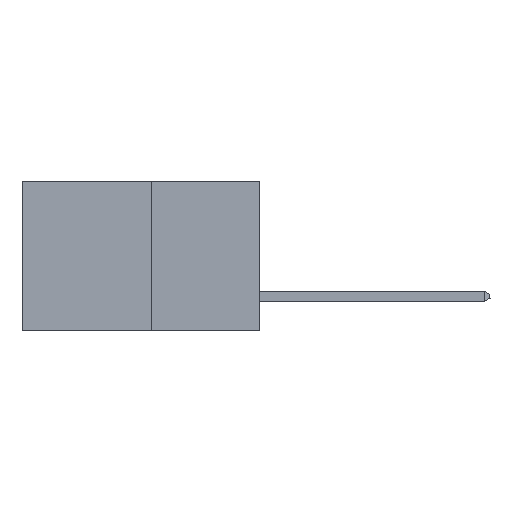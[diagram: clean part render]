
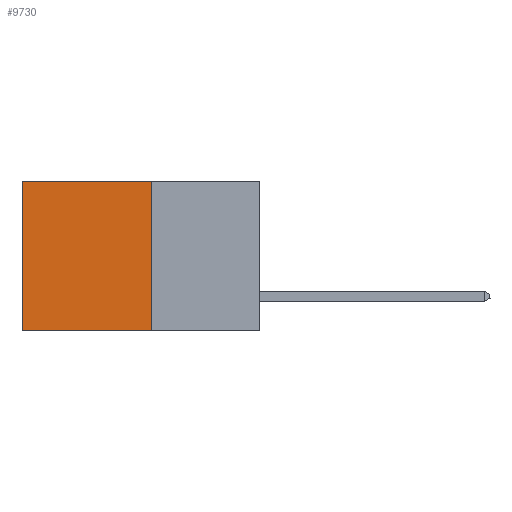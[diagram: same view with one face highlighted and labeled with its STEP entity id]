
A CAD part, left-side view. The second image highlights one B-rep face of the part: STEP entity #9730.
In plain terms, the highlighted planar face has unit normal (-1, 0, 0).
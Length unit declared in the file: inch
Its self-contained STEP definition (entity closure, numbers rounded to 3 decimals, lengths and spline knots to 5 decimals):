
#155 = DIRECTION ( 'NONE',  ( 0., 1., 0. ) ) ;
#170 = VERTEX_POINT ( 'NONE', #330 ) ;
#330 = CARTESIAN_POINT ( 'NONE',  ( 0.277, 0.59, -0.37 ) ) ;
#566 = FACE_OUTER_BOUND ( 'NONE', #10602, .T. ) ;
#955 = VECTOR ( 'NONE', #10435, 39.37008 ) ;
#1531 = LINE ( 'NONE', #7736, #13517 ) ;
#1751 = CARTESIAN_POINT ( 'NONE',  ( 0.277, 0.59, 0. ) ) ;
#1821 = ORIENTED_EDGE ( 'NONE', *, *, #8032, .T. ) ;
#2456 = EDGE_CURVE ( 'NONE', #14388, #170, #10186, .T. ) ;
#2959 = CARTESIAN_POINT ( 'NONE',  ( 0.277, 0.27, -0.37 ) ) ;
#2979 = DIRECTION ( 'NONE',  ( 0., 1., 0. ) ) ;
#3115 = LINE ( 'NONE', #12304, #8902 ) ;
#3394 = VERTEX_POINT ( 'NONE', #14742 ) ;
#3771 = VERTEX_POINT ( 'NONE', #8784 ) ;
#3879 = ORIENTED_EDGE ( 'NONE', *, *, #10291, .F. ) ;
#3886 = CARTESIAN_POINT ( 'NONE',  ( 0.277, 0.27, -0.37 ) ) ;
#5059 = DIRECTION ( 'NONE',  ( 0., 0., -1. ) ) ;
#5264 = VECTOR ( 'NONE', #5059, 39.37008 ) ;
#5602 = ORIENTED_EDGE ( 'NONE', *, *, #2456, .T. ) ;
#6443 = PLANE ( 'NONE',  #7658 ) ;
#7596 = DIRECTION ( 'NONE',  ( 0., 0., -1. ) ) ;
#7658 = AXIS2_PLACEMENT_3D ( 'NONE', #2959, #14531, #7596 ) ;
#7736 = CARTESIAN_POINT ( 'NONE',  ( 0.277, 0.27, 0. ) ) ;
#8032 = EDGE_CURVE ( 'NONE', #3394, #14388, #1531, .T. ) ;
#8784 = CARTESIAN_POINT ( 'NONE',  ( 0.277, 0.27, -0.37 ) ) ;
#8902 = VECTOR ( 'NONE', #2979, 39.37008 ) ;
#9730 = ADVANCED_FACE ( 'NONE', ( #566 ), #6443, .F. ) ;
#10186 = LINE ( 'NONE', #10895, #955 ) ;
#10203 = ORIENTED_EDGE ( 'NONE', *, *, #11891, .F. ) ;
#10291 = EDGE_CURVE ( 'NONE', #3394, #3771, #11477, .T. ) ;
#10435 = DIRECTION ( 'NONE',  ( 0., 0., -1. ) ) ;
#10602 = EDGE_LOOP ( 'NONE', ( #5602, #10203, #3879, #1821 ) ) ;
#10895 = CARTESIAN_POINT ( 'NONE',  ( 0.277, 0.59, -0.37 ) ) ;
#11477 = LINE ( 'NONE', #3886, #5264 ) ;
#11891 = EDGE_CURVE ( 'NONE', #3771, #170, #3115, .T. ) ;
#12304 = CARTESIAN_POINT ( 'NONE',  ( 0.277, 0.27, -0.37 ) ) ;
#13517 = VECTOR ( 'NONE', #155, 39.37008 ) ;
#14388 = VERTEX_POINT ( 'NONE', #1751 ) ;
#14531 = DIRECTION ( 'NONE',  ( 1., 0., 0. ) ) ;
#14742 = CARTESIAN_POINT ( 'NONE',  ( 0.277, 0.27, 0. ) ) ;
